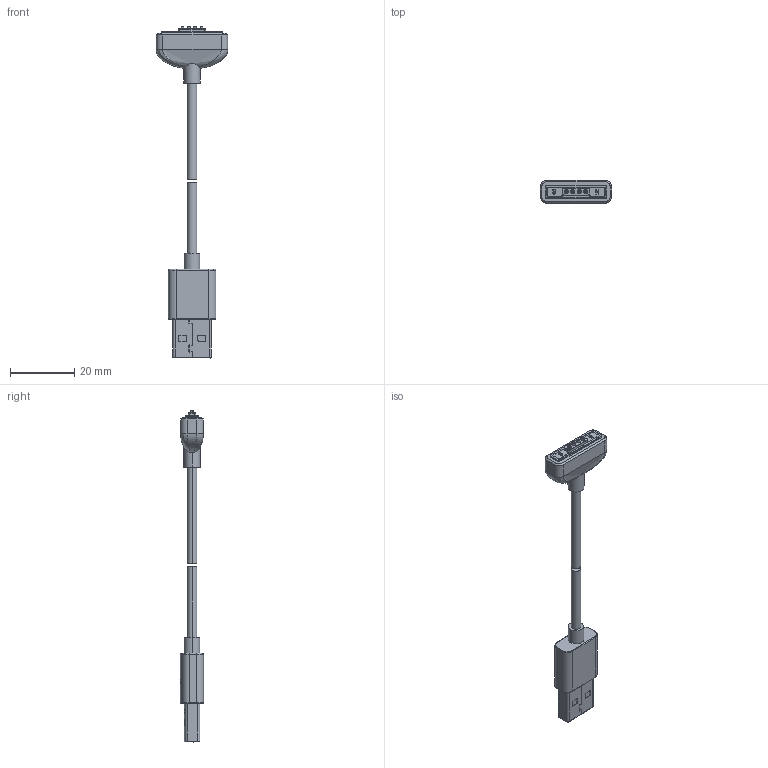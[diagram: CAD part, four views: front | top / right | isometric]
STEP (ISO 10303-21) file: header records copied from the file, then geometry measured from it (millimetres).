
FILE_DESCRIPTION (( 'STEP AP214' ), '1' );
FILE_NAME ('687J0422A511100.STEP', '2023-04-12T19:46:13', ( '' ), ( '' ), 'SwSTEP 2.0', 'SolidWorks 2020', '' );
FILE_SCHEMA (( 'AUTOMOTIVE_DESIGN' ));
Length unit declared in the file: millimetre
Products named in the file (1): 687J0422A511100
Bounding box: 22.3 x 7.17 x 103.4 mm (x, y, z)
Volume: 2986.7 mm3; surface area: 4752.8 mm2
Topology: 2 solids, 7 shells, 1086 faces, 2847 edges, 1774 vertices
Faces by surface type: plane 573, cylinder 333, bspline 106, cone 38, torus 28, sphere 8
Entity records: 52509 total; most frequent: CARTESIAN_POINT 15395, ORIENTED_EDGE 5650, DIRECTION 4623, EDGE_CURVE 2825, VERTEX_POINT 1774, AXIS2_PLACEMENT_3D 1607, LINE 1409, VECTOR 1409
